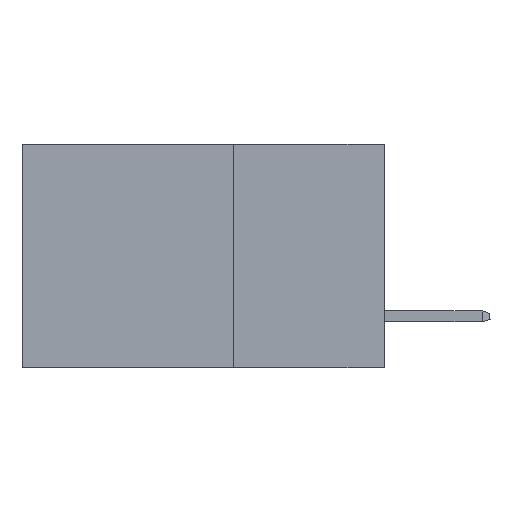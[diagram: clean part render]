
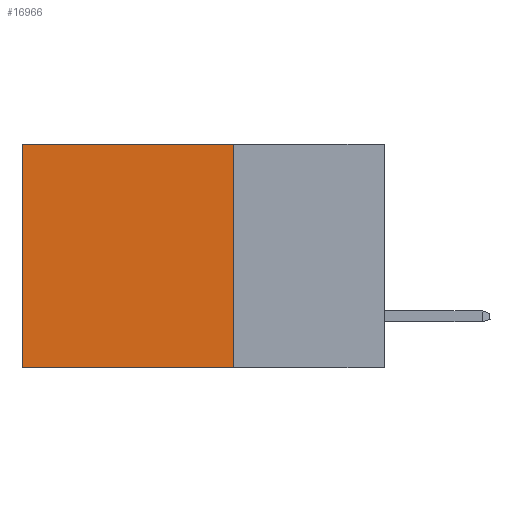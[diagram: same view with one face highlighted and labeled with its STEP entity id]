
A CAD part, left-side view. The second image highlights one B-rep face of the part: STEP entity #16966.
In plain terms, the highlighted planar face has unit normal (-1, 0, 0).
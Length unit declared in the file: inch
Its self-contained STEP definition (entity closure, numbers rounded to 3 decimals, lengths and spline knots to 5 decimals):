
#176 = CARTESIAN_POINT ( 'NONE',  ( 0.298, 0.6, -0.37 ) ) ;
#209 = CARTESIAN_POINT ( 'NONE',  ( 0.298, 0.25, 0. ) ) ;
#1247 = EDGE_CURVE ( 'NONE', #7237, #4622, #20714, .T. ) ;
#1659 = LINE ( 'NONE', #12624, #9767 ) ;
#1667 = DIRECTION ( 'NONE',  ( 0., 0., -1. ) ) ;
#1827 = CARTESIAN_POINT ( 'NONE',  ( 0.298, 0.25, 0. ) ) ;
#3874 = CARTESIAN_POINT ( 'NONE',  ( 0.298, 0.25, -0.37 ) ) ;
#4622 = VERTEX_POINT ( 'NONE', #3874 ) ;
#4917 = EDGE_CURVE ( 'NONE', #4622, #22910, #4947, .T. ) ;
#4947 = LINE ( 'NONE', #6437, #11318 ) ;
#5750 = VERTEX_POINT ( 'NONE', #15269 ) ;
#6104 = DIRECTION ( 'NONE',  ( 1., 0., 0. ) ) ;
#6423 = CARTESIAN_POINT ( 'NONE',  ( 0.298, 0.25, 0. ) ) ;
#6437 = CARTESIAN_POINT ( 'NONE',  ( 0.298, 0.25, -0.37 ) ) ;
#7237 = VERTEX_POINT ( 'NONE', #209 ) ;
#7469 = EDGE_CURVE ( 'NONE', #5750, #22910, #21969, .T. ) ;
#8620 = EDGE_LOOP ( 'NONE', ( #18496, #9313, #17816, #9419 ) ) ;
#9313 = ORIENTED_EDGE ( 'NONE', *, *, #4917, .F. ) ;
#9419 = ORIENTED_EDGE ( 'NONE', *, *, #19950, .T. ) ;
#9767 = VECTOR ( 'NONE', #21993, 39.37008 ) ;
#11318 = VECTOR ( 'NONE', #17597, 39.37008 ) ;
#11817 = PLANE ( 'NONE',  #19720 ) ;
#12624 = CARTESIAN_POINT ( 'NONE',  ( 0.298, 0.25, 0. ) ) ;
#15269 = CARTESIAN_POINT ( 'NONE',  ( 0.298, 0.6, 0. ) ) ;
#16966 = ADVANCED_FACE ( 'NONE', ( #19415 ), #11817, .F. ) ;
#17597 = DIRECTION ( 'NONE',  ( 0., 1., 0. ) ) ;
#17816 = ORIENTED_EDGE ( 'NONE', *, *, #1247, .F. ) ;
#18496 = ORIENTED_EDGE ( 'NONE', *, *, #7469, .T. ) ;
#19024 = DIRECTION ( 'NONE',  ( 0., 0., -1. ) ) ;
#19415 = FACE_OUTER_BOUND ( 'NONE', #8620, .T. ) ;
#19720 = AXIS2_PLACEMENT_3D ( 'NONE', #6423, #6104, #19024 ) ;
#19950 = EDGE_CURVE ( 'NONE', #7237, #5750, #1659, .T. ) ;
#20714 = LINE ( 'NONE', #1827, #23572 ) ;
#20775 = DIRECTION ( 'NONE',  ( 0., 0., -1. ) ) ;
#21969 = LINE ( 'NONE', #22785, #23412 ) ;
#21993 = DIRECTION ( 'NONE',  ( 0., 1., 0. ) ) ;
#22785 = CARTESIAN_POINT ( 'NONE',  ( 0.298, 0.6, 0. ) ) ;
#22910 = VERTEX_POINT ( 'NONE', #176 ) ;
#23412 = VECTOR ( 'NONE', #20775, 39.37008 ) ;
#23572 = VECTOR ( 'NONE', #1667, 39.37008 ) ;
